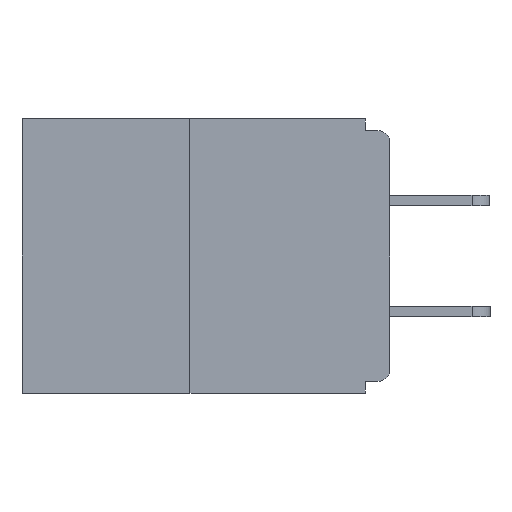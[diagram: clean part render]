
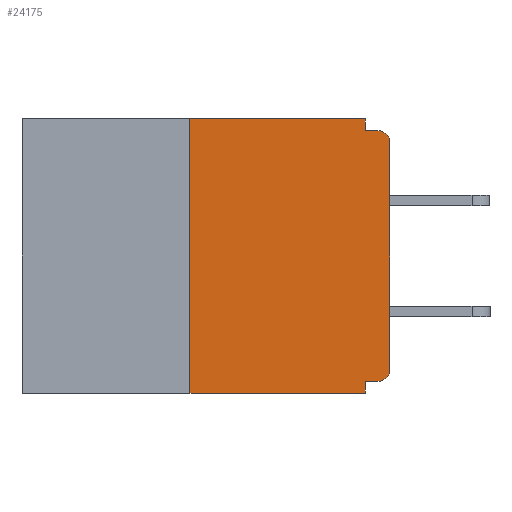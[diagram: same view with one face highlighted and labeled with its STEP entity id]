
A CAD part, left-side view. The second image highlights one B-rep face of the part: STEP entity #24175.
In plain terms, the highlighted planar face has unit normal (-1, 0, 0).
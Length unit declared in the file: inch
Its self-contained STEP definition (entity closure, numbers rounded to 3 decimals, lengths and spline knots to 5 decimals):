
#268 = CARTESIAN_POINT ( 'NONE',  ( 0., 0.25, 0. ) ) ;
#483 = LINE ( 'NONE', #17855, #25491 ) ;
#760 = EDGE_LOOP ( 'NONE', ( #17759, #31088, #23125, #13917, #8002, #19751, #17143, #23261, #20153, #16486 ) ) ;
#1439 = DIRECTION ( 'NONE',  ( -1., 0., 0. ) ) ;
#2580 = EDGE_CURVE ( 'NONE', #9085, #25095, #28639, .T. ) ;
#2682 = DIRECTION ( 'NONE',  ( 0., 0., 1. ) ) ;
#3218 = DIRECTION ( 'NONE',  ( 0., 0., -1. ) ) ;
#4225 = LINE ( 'NONE', #29621, #16318 ) ;
#4524 = VERTEX_POINT ( 'NONE', #27942 ) ;
#4773 = DIRECTION ( 'NONE',  ( 0., 0., -1. ) ) ;
#5203 = EDGE_CURVE ( 'NONE', #30125, #26709, #29568, .T. ) ;
#5569 = CARTESIAN_POINT ( 'NONE',  ( 0., 0.46, 0. ) ) ;
#6840 = EDGE_CURVE ( 'NONE', #30125, #4524, #31263, .T. ) ;
#7098 = CARTESIAN_POINT ( 'NONE',  ( 0., 0., -0.015 ) ) ;
#7338 = CARTESIAN_POINT ( 'NONE',  ( 0., 0.031, 0. ) ) ;
#7858 = VECTOR ( 'NONE', #4773, 39.37008 ) ;
#7952 = VECTOR ( 'NONE', #9568, 39.37008 ) ;
#8002 = ORIENTED_EDGE ( 'NONE', *, *, #6840, .F. ) ;
#8028 = DIRECTION ( 'NONE',  ( 1., 0., 0. ) ) ;
#8274 = VECTOR ( 'NONE', #16096, 39.37008 ) ;
#8727 = CARTESIAN_POINT ( 'NONE',  ( 0., 0.031, -0.015 ) ) ;
#9085 = VERTEX_POINT ( 'NONE', #268 ) ;
#9562 = CIRCLE ( 'NONE', #24584, 0.015 ) ;
#9568 = DIRECTION ( 'NONE',  ( 0., -1., 0. ) ) ;
#10263 = EDGE_CURVE ( 'NONE', #22207, #29556, #9562, .T. ) ;
#10461 = FACE_OUTER_BOUND ( 'NONE', #760, .T. ) ;
#11017 = DIRECTION ( 'NONE',  ( 0., 0., -1. ) ) ;
#11171 = EDGE_CURVE ( 'NONE', #26163, #9085, #11412, .T. ) ;
#11412 = LINE ( 'NONE', #28220, #13971 ) ;
#11605 = CARTESIAN_POINT ( 'NONE',  ( 0., 0.031, -0.343 ) ) ;
#12122 = CARTESIAN_POINT ( 'NONE',  ( 0., 0., -0.03 ) ) ;
#12352 = DIRECTION ( 'NONE',  ( 0., 1., 0. ) ) ;
#13917 = ORIENTED_EDGE ( 'NONE', *, *, #19767, .F. ) ;
#13971 = VECTOR ( 'NONE', #18501, 39.37008 ) ;
#14473 = CARTESIAN_POINT ( 'NONE',  ( 0., 0.031, -0.343 ) ) ;
#14543 = CARTESIAN_POINT ( 'NONE',  ( 0., 0., -0.328 ) ) ;
#14812 = CARTESIAN_POINT ( 'NONE',  ( 0., 0.015, -0.015 ) ) ;
#15174 = PLANE ( 'NONE',  #17967 ) ;
#15375 = EDGE_CURVE ( 'NONE', #26709, #22207, #4225, .T. ) ;
#16096 = DIRECTION ( 'NONE',  ( 0., -1., 0. ) ) ;
#16318 = VECTOR ( 'NONE', #2682, 39.37008 ) ;
#16486 = ORIENTED_EDGE ( 'NONE', *, *, #23275, .F. ) ;
#17039 = CARTESIAN_POINT ( 'NONE',  ( 0., 0., -0.313 ) ) ;
#17143 = ORIENTED_EDGE ( 'NONE', *, *, #15375, .T. ) ;
#17759 = ORIENTED_EDGE ( 'NONE', *, *, #2580, .F. ) ;
#17855 = CARTESIAN_POINT ( 'NONE',  ( 0., 0.46, -0.343 ) ) ;
#17967 = AXIS2_PLACEMENT_3D ( 'NONE', #5569, #8028, #3218 ) ;
#18179 = DIRECTION ( 'NONE',  ( 0., -1., 0. ) ) ;
#18501 = DIRECTION ( 'NONE',  ( 0., 0., 1. ) ) ;
#19481 = EDGE_CURVE ( 'NONE', #26163, #29387, #483, .T. ) ;
#19751 = ORIENTED_EDGE ( 'NONE', *, *, #5203, .T. ) ;
#19767 = EDGE_CURVE ( 'NONE', #4524, #29387, #25826, .T. ) ;
#20003 = CARTESIAN_POINT ( 'NONE',  ( 0., 0.015, -0.328 ) ) ;
#20153 = ORIENTED_EDGE ( 'NONE', *, *, #27157, .F. ) ;
#20367 = CARTESIAN_POINT ( 'NONE',  ( 0., 0.015, -0.313 ) ) ;
#20775 = LINE ( 'NONE', #7098, #7952 ) ;
#21595 = DIRECTION ( 'NONE',  ( 0., 0., -1. ) ) ;
#22207 = VERTEX_POINT ( 'NONE', #12122 ) ;
#22297 = DIRECTION ( 'NONE',  ( -1., 0., 0. ) ) ;
#22402 = DIRECTION ( 'NONE',  ( 0., 0., -1. ) ) ;
#23125 = ORIENTED_EDGE ( 'NONE', *, *, #19481, .T. ) ;
#23261 = ORIENTED_EDGE ( 'NONE', *, *, #10263, .T. ) ;
#23275 = EDGE_CURVE ( 'NONE', #25095, #26921, #26764, .T. ) ;
#23484 = AXIS2_PLACEMENT_3D ( 'NONE', #20367, #1439, #11017 ) ;
#24175 = ADVANCED_FACE ( 'NONE', ( #10461 ), #15174, .F. ) ;
#24298 = CARTESIAN_POINT ( 'NONE',  ( 0., 0.031, 0. ) ) ;
#24584 = AXIS2_PLACEMENT_3D ( 'NONE', #24749, #22297, #22402 ) ;
#24708 = VECTOR ( 'NONE', #21595, 39.37008 ) ;
#24749 = CARTESIAN_POINT ( 'NONE',  ( 0., 0.015, -0.03 ) ) ;
#25095 = VERTEX_POINT ( 'NONE', #24298 ) ;
#25491 = VECTOR ( 'NONE', #18179, 39.37008 ) ;
#25613 = VECTOR ( 'NONE', #12352, 39.37008 ) ;
#25826 = LINE ( 'NONE', #11605, #24708 ) ;
#26163 = VERTEX_POINT ( 'NONE', #28706 ) ;
#26709 = VERTEX_POINT ( 'NONE', #17039 ) ;
#26764 = LINE ( 'NONE', #7338, #7858 ) ;
#26921 = VERTEX_POINT ( 'NONE', #8727 ) ;
#27157 = EDGE_CURVE ( 'NONE', #26921, #29556, #20775, .T. ) ;
#27942 = CARTESIAN_POINT ( 'NONE',  ( 0., 0.031, -0.328 ) ) ;
#28220 = CARTESIAN_POINT ( 'NONE',  ( 0., 0.25, 0. ) ) ;
#28639 = LINE ( 'NONE', #30981, #8274 ) ;
#28706 = CARTESIAN_POINT ( 'NONE',  ( 0., 0.25, -0.343 ) ) ;
#29387 = VERTEX_POINT ( 'NONE', #14473 ) ;
#29556 = VERTEX_POINT ( 'NONE', #14812 ) ;
#29568 = CIRCLE ( 'NONE', #23484, 0.015 ) ;
#29621 = CARTESIAN_POINT ( 'NONE',  ( 0., 0., 0. ) ) ;
#30125 = VERTEX_POINT ( 'NONE', #20003 ) ;
#30981 = CARTESIAN_POINT ( 'NONE',  ( 0., 0.46, 0. ) ) ;
#31088 = ORIENTED_EDGE ( 'NONE', *, *, #11171, .F. ) ;
#31263 = LINE ( 'NONE', #14543, #25613 ) ;
